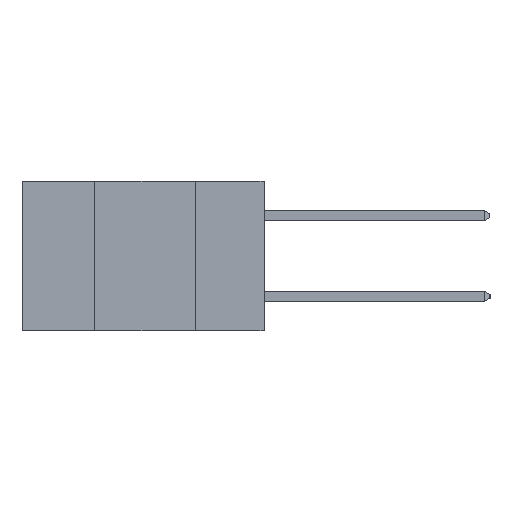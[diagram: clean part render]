
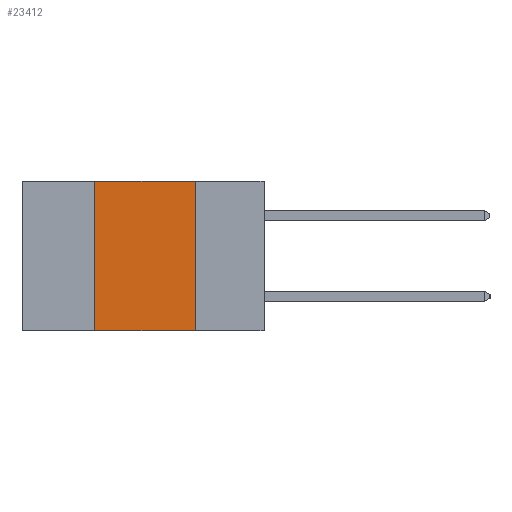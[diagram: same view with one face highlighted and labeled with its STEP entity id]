
A CAD part, left-side view. The second image highlights one B-rep face of the part: STEP entity #23412.
In plain terms, the highlighted planar face has unit normal (-1, 0, 0).
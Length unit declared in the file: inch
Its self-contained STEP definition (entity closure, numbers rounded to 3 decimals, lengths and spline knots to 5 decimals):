
#1047 = FACE_OUTER_BOUND ( 'NONE', #22699, .T. ) ;
#2367 = LINE ( 'NONE', #24058, #13682 ) ;
#2747 = DIRECTION ( 'NONE',  ( 0., -1., 0. ) ) ;
#3254 = CARTESIAN_POINT ( 'NONE',  ( 0., 0.42, 0. ) ) ;
#3286 = VERTEX_POINT ( 'NONE', #3254 ) ;
#3436 = VERTEX_POINT ( 'NONE', #18575 ) ;
#3782 = VERTEX_POINT ( 'NONE', #4883 ) ;
#4883 = CARTESIAN_POINT ( 'NONE',  ( 0., 0.17, -0.37 ) ) ;
#4976 = LINE ( 'NONE', #17602, #26732 ) ;
#5292 = DIRECTION ( 'NONE',  ( 0., 0., -1. ) ) ;
#6240 = LINE ( 'NONE', #7288, #7581 ) ;
#7128 = DIRECTION ( 'NONE',  ( 0., -1., 0. ) ) ;
#7284 = ORIENTED_EDGE ( 'NONE', *, *, #17617, .F. ) ;
#7288 = CARTESIAN_POINT ( 'NONE',  ( 0., 0.17, -0.37 ) ) ;
#7331 = VECTOR ( 'NONE', #10885, 39.37008 ) ;
#7581 = VECTOR ( 'NONE', #22111, 39.37008 ) ;
#7625 = EDGE_CURVE ( 'NONE', #3436, #3782, #2367, .T. ) ;
#8261 = CARTESIAN_POINT ( 'NONE',  ( 0., 0.17, 0. ) ) ;
#10885 = DIRECTION ( 'NONE',  ( 0., 0., 1. ) ) ;
#11618 = ORIENTED_EDGE ( 'NONE', *, *, #19038, .F. ) ;
#12512 = VERTEX_POINT ( 'NONE', #8261 ) ;
#12994 = LINE ( 'NONE', #25599, #7331 ) ;
#13682 = VECTOR ( 'NONE', #7128, 39.37008 ) ;
#13777 = PLANE ( 'NONE',  #18147 ) ;
#15913 = CARTESIAN_POINT ( 'NONE',  ( 0., 0.6, 0. ) ) ;
#16197 = EDGE_CURVE ( 'NONE', #3436, #3286, #12994, .T. ) ;
#17602 = CARTESIAN_POINT ( 'NONE',  ( 0., 0.6, 0. ) ) ;
#17617 = EDGE_CURVE ( 'NONE', #3286, #12512, #4976, .T. ) ;
#18037 = DIRECTION ( 'NONE',  ( 1., 0., 0. ) ) ;
#18147 = AXIS2_PLACEMENT_3D ( 'NONE', #15913, #18037, #5292 ) ;
#18575 = CARTESIAN_POINT ( 'NONE',  ( 0., 0.42, -0.37 ) ) ;
#19038 = EDGE_CURVE ( 'NONE', #12512, #3782, #6240, .T. ) ;
#20958 = ORIENTED_EDGE ( 'NONE', *, *, #7625, .T. ) ;
#22111 = DIRECTION ( 'NONE',  ( 0., 0., -1. ) ) ;
#22699 = EDGE_LOOP ( 'NONE', ( #11618, #7284, #24804, #20958 ) ) ;
#23412 = ADVANCED_FACE ( 'NONE', ( #1047 ), #13777, .F. ) ;
#24058 = CARTESIAN_POINT ( 'NONE',  ( 0., 0.6, -0.37 ) ) ;
#24804 = ORIENTED_EDGE ( 'NONE', *, *, #16197, .F. ) ;
#25599 = CARTESIAN_POINT ( 'NONE',  ( 0., 0.42, -0.37 ) ) ;
#26732 = VECTOR ( 'NONE', #2747, 39.37008 ) ;
